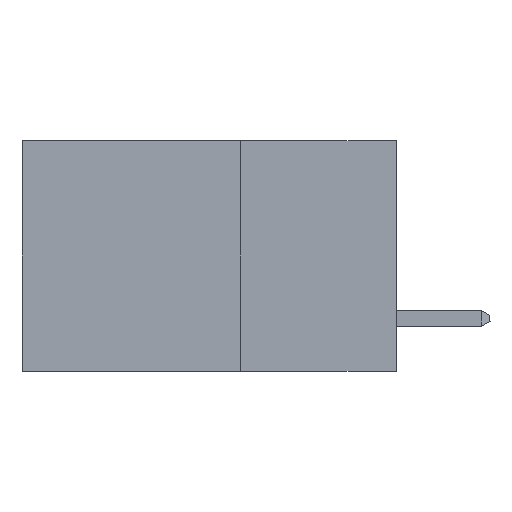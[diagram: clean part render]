
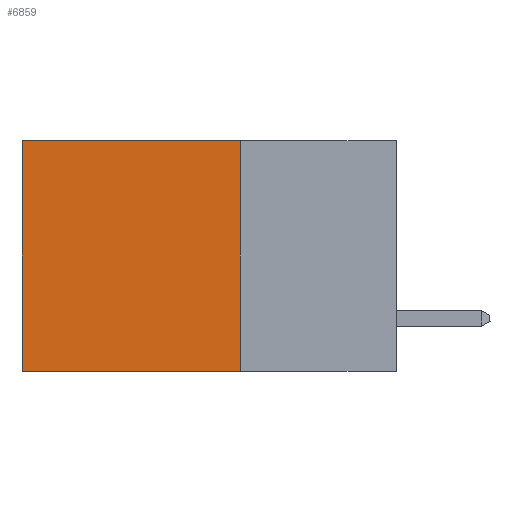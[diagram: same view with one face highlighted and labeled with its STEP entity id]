
A CAD part, left-side view. The second image highlights one B-rep face of the part: STEP entity #6859.
In plain terms, the highlighted planar face has unit normal (-1, 0, 0).
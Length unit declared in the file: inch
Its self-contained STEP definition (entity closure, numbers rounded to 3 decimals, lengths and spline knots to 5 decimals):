
#127 = AXIS2_PLACEMENT_3D ( 'NONE', #5587, #6849, #14883 ) ;
#161 = EDGE_CURVE ( 'NONE', #15548, #15736, #7464, .T. ) ;
#377 = CARTESIAN_POINT ( 'NONE',  ( 0.298, 0.25, 0. ) ) ;
#621 = VERTEX_POINT ( 'NONE', #4613 ) ;
#1667 = LINE ( 'NONE', #6607, #15245 ) ;
#1919 = EDGE_CURVE ( 'NONE', #15548, #2453, #1667, .T. ) ;
#2453 = VERTEX_POINT ( 'NONE', #9279 ) ;
#2820 = DIRECTION ( 'NONE',  ( 0., 0., -1. ) ) ;
#3229 = CARTESIAN_POINT ( 'NONE',  ( 0.298, 0.6, 0. ) ) ;
#3923 = VECTOR ( 'NONE', #10368, 39.37008 ) ;
#3994 = DIRECTION ( 'NONE',  ( 0., 1., 0. ) ) ;
#4613 = CARTESIAN_POINT ( 'NONE',  ( 0.298, 0.6, -0.37 ) ) ;
#4774 = DIRECTION ( 'NONE',  ( 0., 0., -1. ) ) ;
#5185 = CARTESIAN_POINT ( 'NONE',  ( 0.298, 0.6, 0. ) ) ;
#5587 = CARTESIAN_POINT ( 'NONE',  ( 0.298, 0.25, 0. ) ) ;
#6607 = CARTESIAN_POINT ( 'NONE',  ( 0.298, 0.25, 0. ) ) ;
#6849 = DIRECTION ( 'NONE',  ( 1., 0., 0. ) ) ;
#6859 = ADVANCED_FACE ( 'NONE', ( #15805 ), #6901, .F. ) ;
#6901 = PLANE ( 'NONE',  #127 ) ;
#7396 = LINE ( 'NONE', #11643, #3923 ) ;
#7464 = LINE ( 'NONE', #7883, #10535 ) ;
#7883 = CARTESIAN_POINT ( 'NONE',  ( 0.298, 0.25, 0. ) ) ;
#8315 = VECTOR ( 'NONE', #4774, 39.37008 ) ;
#8369 = EDGE_LOOP ( 'NONE', ( #11130, #10555, #11275, #9453 ) ) ;
#9033 = EDGE_CURVE ( 'NONE', #15736, #621, #16571, .T. ) ;
#9279 = CARTESIAN_POINT ( 'NONE',  ( 0.298, 0.25, -0.37 ) ) ;
#9453 = ORIENTED_EDGE ( 'NONE', *, *, #161, .T. ) ;
#10368 = DIRECTION ( 'NONE',  ( 0., 1., 0. ) ) ;
#10535 = VECTOR ( 'NONE', #3994, 39.37008 ) ;
#10555 = ORIENTED_EDGE ( 'NONE', *, *, #16725, .F. ) ;
#11130 = ORIENTED_EDGE ( 'NONE', *, *, #9033, .T. ) ;
#11275 = ORIENTED_EDGE ( 'NONE', *, *, #1919, .F. ) ;
#11643 = CARTESIAN_POINT ( 'NONE',  ( 0.298, 0.25, -0.37 ) ) ;
#14883 = DIRECTION ( 'NONE',  ( 0., 0., -1. ) ) ;
#15245 = VECTOR ( 'NONE', #2820, 39.37008 ) ;
#15548 = VERTEX_POINT ( 'NONE', #377 ) ;
#15736 = VERTEX_POINT ( 'NONE', #5185 ) ;
#15805 = FACE_OUTER_BOUND ( 'NONE', #8369, .T. ) ;
#16571 = LINE ( 'NONE', #3229, #8315 ) ;
#16725 = EDGE_CURVE ( 'NONE', #2453, #621, #7396, .T. ) ;
